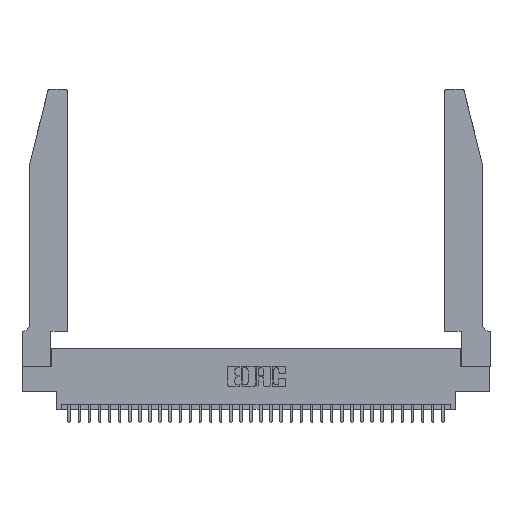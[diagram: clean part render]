
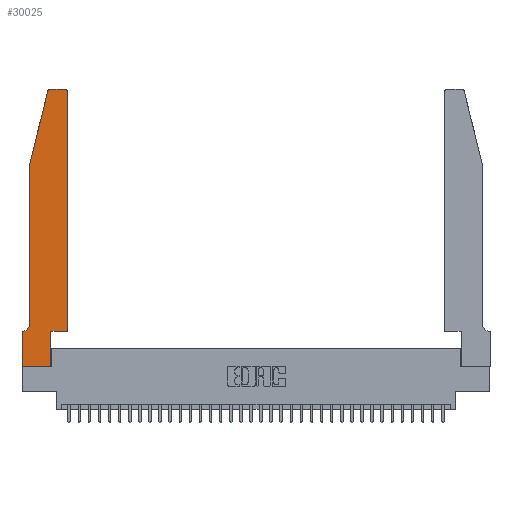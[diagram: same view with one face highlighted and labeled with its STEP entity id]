
A CAD part, top view. The second image highlights one B-rep face of the part: STEP entity #30025.
In plain terms, the highlighted planar face has unit normal (0, 0, 1).
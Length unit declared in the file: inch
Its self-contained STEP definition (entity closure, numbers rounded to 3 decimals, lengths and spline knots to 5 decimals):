
#348 = VERTEX_POINT ( 'NONE', #29483 ) ;
#520 = EDGE_CURVE ( 'NONE', #15657, #4800, #15304, .T. ) ;
#866 = DIRECTION ( 'NONE',  ( 0., 0., -1. ) ) ;
#976 = DIRECTION ( 'NONE',  ( 0., 0., 1. ) ) ;
#1009 = DIRECTION ( 'NONE',  ( 1., 0., 0. ) ) ;
#1655 = EDGE_CURVE ( 'NONE', #11825, #348, #3236, .T. ) ;
#2430 = EDGE_CURVE ( 'NONE', #4833, #20259, #24109, .T. ) ;
#3087 = VECTOR ( 'NONE', #9478, 39.37008 ) ;
#3236 = CIRCLE ( 'NONE', #27946, 0.03 ) ;
#4400 = CARTESIAN_POINT ( 'NONE',  ( 0.4505, 0.35, 0.37 ) ) ;
#4800 = VERTEX_POINT ( 'NONE', #4400 ) ;
#4833 = VERTEX_POINT ( 'NONE', #7974 ) ;
#5334 = VECTOR ( 'NONE', #15170, 39.37008 ) ;
#5348 = ORIENTED_EDGE ( 'NONE', *, *, #10526, .T. ) ;
#6255 = CARTESIAN_POINT ( 'NONE',  ( 0., 0., 0.37 ) ) ;
#6341 = CARTESIAN_POINT ( 'NONE',  ( 0., 0.35, 0.37 ) ) ;
#6566 = DIRECTION ( 'NONE',  ( 0., 1., 0. ) ) ;
#6585 = DIRECTION ( 'NONE',  ( -1., 0., 0. ) ) ;
#7507 = LINE ( 'NONE', #6255, #5334 ) ;
#7532 = ORIENTED_EDGE ( 'NONE', *, *, #19512, .T. ) ;
#7974 = CARTESIAN_POINT ( 'NONE',  ( 0.25487, 2.72718, 0.37 ) ) ;
#8072 = VECTOR ( 'NONE', #29440, 39.37008 ) ;
#8679 = LINE ( 'NONE', #20532, #11647 ) ;
#8756 = CARTESIAN_POINT ( 'NONE',  ( 0.0055, 0.35, 0.37 ) ) ;
#8870 = CARTESIAN_POINT ( 'NONE',  ( 0., 0.35, 0.37 ) ) ;
#9108 = DIRECTION ( 'NONE',  ( 0., 0., 1. ) ) ;
#9309 = DIRECTION ( 'NONE',  ( 1., 0., 0. ) ) ;
#9478 = DIRECTION ( 'NONE',  ( 0., 1., 0. ) ) ;
#9604 = LINE ( 'NONE', #11450, #35174 ) ;
#9746 = VERTEX_POINT ( 'NONE', #8870 ) ;
#10339 = CARTESIAN_POINT ( 'NONE',  ( 0.0755, 0.42, 0.37 ) ) ;
#10526 = EDGE_CURVE ( 'NONE', #348, #22012, #22990, .T. ) ;
#10883 = EDGE_CURVE ( 'NONE', #9746, #33487, #22963, .T. ) ;
#11450 = CARTESIAN_POINT ( 'NONE',  ( 0.4505, 0.35, 0.37 ) ) ;
#11647 = VECTOR ( 'NONE', #19370, 39.37008 ) ;
#11825 = VERTEX_POINT ( 'NONE', #16038 ) ;
#12134 = EDGE_CURVE ( 'NONE', #33487, #34881, #7507, .T. ) ;
#12737 = CARTESIAN_POINT ( 'NONE',  ( 0.0755, 0.35, 0.37 ) ) ;
#13041 = DIRECTION ( 'NONE',  ( -1., 0., 0. ) ) ;
#13662 = AXIS2_PLACEMENT_3D ( 'NONE', #27555, #866, #6585 ) ;
#14006 = ORIENTED_EDGE ( 'NONE', *, *, #1655, .T. ) ;
#14187 = CARTESIAN_POINT ( 'NONE',  ( 0.284, 2.72, 0.37 ) ) ;
#14205 = CARTESIAN_POINT ( 'NONE',  ( 0., 0., 0.37 ) ) ;
#15170 = DIRECTION ( 'NONE',  ( 1., 0., 0. ) ) ;
#15304 = LINE ( 'NONE', #34322, #8072 ) ;
#15591 = VECTOR ( 'NONE', #34796, 39.37008 ) ;
#15657 = VERTEX_POINT ( 'NONE', #23401 ) ;
#16038 = CARTESIAN_POINT ( 'NONE',  ( 0.4505, 2.72, 0.37 ) ) ;
#16098 = FACE_OUTER_BOUND ( 'NONE', #30355, .T. ) ;
#16434 = LINE ( 'NONE', #12737, #15591 ) ;
#16476 = AXIS2_PLACEMENT_3D ( 'NONE', #14187, #16941, #32909 ) ;
#16941 = DIRECTION ( 'NONE',  ( 0., 0., 1. ) ) ;
#17531 = PLANE ( 'NONE',  #24918 ) ;
#17653 = EDGE_CURVE ( 'NONE', #34881, #15657, #21021, .T. ) ;
#18622 = DIRECTION ( 'NONE',  ( 0., -1., 0. ) ) ;
#19370 = DIRECTION ( 'NONE',  ( 0., -1., 0. ) ) ;
#19499 = EDGE_CURVE ( 'NONE', #20259, #21072, #8679, .T. ) ;
#19512 = EDGE_CURVE ( 'NONE', #21072, #29507, #23606, .T. ) ;
#20259 = VERTEX_POINT ( 'NONE', #30781 ) ;
#20423 = VECTOR ( 'NONE', #13041, 39.37008 ) ;
#20532 = CARTESIAN_POINT ( 'NONE',  ( 0.0755, 2., 0.37 ) ) ;
#21021 = LINE ( 'NONE', #23546, #3087 ) ;
#21072 = VERTEX_POINT ( 'NONE', #10339 ) ;
#21182 = CARTESIAN_POINT ( 'NONE',  ( 0.2605, 2.75, 0.37 ) ) ;
#21703 = CARTESIAN_POINT ( 'NONE',  ( 0., 0., 0.37 ) ) ;
#22012 = VERTEX_POINT ( 'NONE', #28977 ) ;
#22963 = LINE ( 'NONE', #21703, #31053 ) ;
#22990 = LINE ( 'NONE', #21182, #20423 ) ;
#23092 = EDGE_CURVE ( 'NONE', #22012, #4833, #35276, .T. ) ;
#23401 = CARTESIAN_POINT ( 'NONE',  ( 0.2865, 0.35, 0.37 ) ) ;
#23546 = CARTESIAN_POINT ( 'NONE',  ( 0.2865, 0.35, 0.37 ) ) ;
#23606 = CIRCLE ( 'NONE', #13662, 0.07 ) ;
#23650 = ORIENTED_EDGE ( 'NONE', *, *, #10883, .T. ) ;
#24109 = LINE ( 'NONE', #26191, #32608 ) ;
#24278 = EDGE_CURVE ( 'NONE', #29507, #9746, #16434, .T. ) ;
#24918 = AXIS2_PLACEMENT_3D ( 'NONE', #6341, #976, #9309 ) ;
#25436 = CARTESIAN_POINT ( 'NONE',  ( 0.4205, 2.72, 0.37 ) ) ;
#26042 = CARTESIAN_POINT ( 'NONE',  ( 0.2865, 0., 0.37 ) ) ;
#26191 = CARTESIAN_POINT ( 'NONE',  ( 0.0755, 2., 0.37 ) ) ;
#27066 = ORIENTED_EDGE ( 'NONE', *, *, #19499, .T. ) ;
#27555 = CARTESIAN_POINT ( 'NONE',  ( 0.0055, 0.42, 0.37 ) ) ;
#27946 = AXIS2_PLACEMENT_3D ( 'NONE', #25436, #9108, #1009 ) ;
#28543 = ORIENTED_EDGE ( 'NONE', *, *, #12134, .T. ) ;
#28977 = CARTESIAN_POINT ( 'NONE',  ( 0.284, 2.75, 0.37 ) ) ;
#29061 = DIRECTION ( 'NONE',  ( -0.239, -0.971, 0. ) ) ;
#29440 = DIRECTION ( 'NONE',  ( 1., 0., 0. ) ) ;
#29483 = CARTESIAN_POINT ( 'NONE',  ( 0.4205, 2.75, 0.37 ) ) ;
#29507 = VERTEX_POINT ( 'NONE', #8756 ) ;
#30025 = ADVANCED_FACE ( 'NONE', ( #16098 ), #17531, .T. ) ;
#30309 = ORIENTED_EDGE ( 'NONE', *, *, #17653, .T. ) ;
#30355 = EDGE_LOOP ( 'NONE', ( #5348, #32921, #32182, #27066, #7532, #32173, #23650, #28543, #30309, #31750, #30415, #14006 ) ) ;
#30415 = ORIENTED_EDGE ( 'NONE', *, *, #34122, .T. ) ;
#30781 = CARTESIAN_POINT ( 'NONE',  ( 0.0755, 2., 0.37 ) ) ;
#31053 = VECTOR ( 'NONE', #18622, 39.37008 ) ;
#31750 = ORIENTED_EDGE ( 'NONE', *, *, #520, .T. ) ;
#32173 = ORIENTED_EDGE ( 'NONE', *, *, #24278, .T. ) ;
#32182 = ORIENTED_EDGE ( 'NONE', *, *, #2430, .T. ) ;
#32608 = VECTOR ( 'NONE', #29061, 39.37008 ) ;
#32909 = DIRECTION ( 'NONE',  ( 1., 0., 0. ) ) ;
#32921 = ORIENTED_EDGE ( 'NONE', *, *, #23092, .T. ) ;
#33487 = VERTEX_POINT ( 'NONE', #14205 ) ;
#34122 = EDGE_CURVE ( 'NONE', #4800, #11825, #9604, .T. ) ;
#34322 = CARTESIAN_POINT ( 'NONE',  ( 0.4505, 0.35, 0.37 ) ) ;
#34796 = DIRECTION ( 'NONE',  ( -1., 0., 0. ) ) ;
#34881 = VERTEX_POINT ( 'NONE', #26042 ) ;
#35174 = VECTOR ( 'NONE', #6566, 39.37008 ) ;
#35276 = CIRCLE ( 'NONE', #16476, 0.03 ) ;
